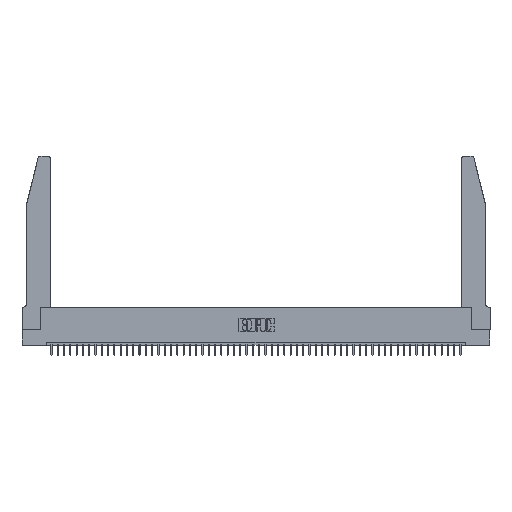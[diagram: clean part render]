
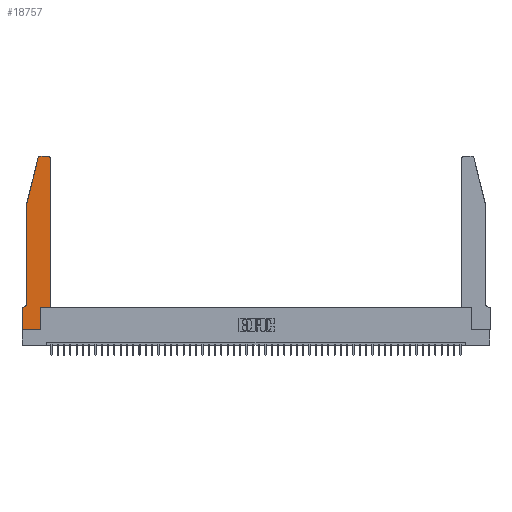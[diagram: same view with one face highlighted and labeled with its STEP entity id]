
A CAD part, top view. The second image highlights one B-rep face of the part: STEP entity #18757.
In plain terms, the highlighted planar face has unit normal (0, 0, 1).
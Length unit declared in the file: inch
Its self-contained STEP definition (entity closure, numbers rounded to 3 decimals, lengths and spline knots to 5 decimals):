
#239 = EDGE_CURVE ( 'NONE', #17133, #3528, #24382, .T. ) ;
#579 = ORIENTED_EDGE ( 'NONE', *, *, #7170, .T. ) ;
#968 = VECTOR ( 'NONE', #34424, 39.37008 ) ;
#1451 = DIRECTION ( 'NONE',  ( 0., -1., 0. ) ) ;
#2596 = ORIENTED_EDGE ( 'NONE', *, *, #239, .T. ) ;
#2757 = EDGE_CURVE ( 'NONE', #3528, #3421, #14084, .T. ) ;
#3236 = ORIENTED_EDGE ( 'NONE', *, *, #50966, .T. ) ;
#3421 = VERTEX_POINT ( 'NONE', #10675 ) ;
#3528 = VERTEX_POINT ( 'NONE', #52247 ) ;
#3619 = CARTESIAN_POINT ( 'NONE',  ( 0.4205, 2.72, 0.37 ) ) ;
#4620 = CARTESIAN_POINT ( 'NONE',  ( 0.2865, 0.35, 0.37 ) ) ;
#5196 = LINE ( 'NONE', #27130, #45272 ) ;
#5522 = CARTESIAN_POINT ( 'NONE',  ( 0.0055, 0.42, 0.37 ) ) ;
#5592 = VECTOR ( 'NONE', #7204, 39.37008 ) ;
#5607 = DIRECTION ( 'NONE',  ( -1., 0., 0. ) ) ;
#5769 = CIRCLE ( 'NONE', #48783, 0.03 ) ;
#6192 = CARTESIAN_POINT ( 'NONE',  ( 0.0755, 2., 0.37 ) ) ;
#6992 = VECTOR ( 'NONE', #36110, 39.37008 ) ;
#7170 = EDGE_CURVE ( 'NONE', #42297, #19794, #5196, .T. ) ;
#7204 = DIRECTION ( 'NONE',  ( 0., 1., 0. ) ) ;
#7736 = EDGE_CURVE ( 'NONE', #19794, #12716, #29137, .T. ) ;
#7805 = DIRECTION ( 'NONE',  ( 1., 0., 0. ) ) ;
#9256 = VERTEX_POINT ( 'NONE', #20116 ) ;
#9715 = DIRECTION ( 'NONE',  ( -1., 0., 0. ) ) ;
#10080 = DIRECTION ( 'NONE',  ( 0., 0., 1. ) ) ;
#10675 = CARTESIAN_POINT ( 'NONE',  ( 0.0755, 0.42, 0.37 ) ) ;
#10941 = CARTESIAN_POINT ( 'NONE',  ( 0.284, 2.72, 0.37 ) ) ;
#12716 = VERTEX_POINT ( 'NONE', #38595 ) ;
#12789 = VECTOR ( 'NONE', #18734, 39.37008 ) ;
#12966 = VECTOR ( 'NONE', #5607, 39.37008 ) ;
#13414 = VECTOR ( 'NONE', #52285, 39.37008 ) ;
#13481 = CARTESIAN_POINT ( 'NONE',  ( 0.4505, 0.35, 0.37 ) ) ;
#14084 = LINE ( 'NONE', #6192, #12789 ) ;
#14980 = AXIS2_PLACEMENT_3D ( 'NONE', #5522, #34498, #9715 ) ;
#15116 = DIRECTION ( 'NONE',  ( 1., 0., 0. ) ) ;
#15310 = EDGE_CURVE ( 'NONE', #9256, #40806, #22647, .T. ) ;
#15938 = CARTESIAN_POINT ( 'NONE',  ( 0., 0.35, 0.37 ) ) ;
#16922 = ORIENTED_EDGE ( 'NONE', *, *, #2757, .T. ) ;
#17133 = VERTEX_POINT ( 'NONE', #32875 ) ;
#18734 = DIRECTION ( 'NONE',  ( 0., -1., 0. ) ) ;
#18757 = ADVANCED_FACE ( 'NONE', ( #24942 ), #26548, .T. ) ;
#19310 = CARTESIAN_POINT ( 'NONE',  ( 0.2865, 0., 0.37 ) ) ;
#19583 = VERTEX_POINT ( 'NONE', #44300 ) ;
#19794 = VERTEX_POINT ( 'NONE', #13481 ) ;
#20116 = CARTESIAN_POINT ( 'NONE',  ( 0.4205, 2.75, 0.37 ) ) ;
#20121 = ORIENTED_EDGE ( 'NONE', *, *, #49427, .T. ) ;
#20726 = ORIENTED_EDGE ( 'NONE', *, *, #30848, .T. ) ;
#21307 = EDGE_LOOP ( 'NONE', ( #24708, #29857, #2596, #16922, #3236, #24000, #20121, #20726, #37521, #579, #32359, #46459 ) ) ;
#21375 = EDGE_CURVE ( 'NONE', #40806, #17133, #5769, .T. ) ;
#22647 = LINE ( 'NONE', #34583, #12966 ) ;
#22753 = DIRECTION ( 'NONE',  ( 0., 1., 0. ) ) ;
#23027 = LINE ( 'NONE', #30447, #43660 ) ;
#23273 = AXIS2_PLACEMENT_3D ( 'NONE', #3619, #32618, #7805 ) ;
#24000 = ORIENTED_EDGE ( 'NONE', *, *, #49415, .T. ) ;
#24382 = LINE ( 'NONE', #35837, #13414 ) ;
#24708 = ORIENTED_EDGE ( 'NONE', *, *, #15310, .T. ) ;
#24942 = FACE_OUTER_BOUND ( 'NONE', #21307, .T. ) ;
#26548 = PLANE ( 'NONE',  #36709 ) ;
#27130 = CARTESIAN_POINT ( 'NONE',  ( 0.4505, 0.35, 0.37 ) ) ;
#27231 = EDGE_CURVE ( 'NONE', #12716, #9256, #37071, .T. ) ;
#27850 = CARTESIAN_POINT ( 'NONE',  ( 0.2865, 0.35, 0.37 ) ) ;
#29137 = LINE ( 'NONE', #35053, #50620 ) ;
#29857 = ORIENTED_EDGE ( 'NONE', *, *, #21375, .T. ) ;
#30281 = CARTESIAN_POINT ( 'NONE',  ( 0.0755, 0.35, 0.37 ) ) ;
#30447 = CARTESIAN_POINT ( 'NONE',  ( 0., 0., 0.37 ) ) ;
#30701 = CARTESIAN_POINT ( 'NONE',  ( 0., 0.35, 0.37 ) ) ;
#30848 = EDGE_CURVE ( 'NONE', #19583, #51218, #52118, .T. ) ;
#31283 = DIRECTION ( 'NONE',  ( 1., 0., 0. ) ) ;
#31354 = VERTEX_POINT ( 'NONE', #43969 ) ;
#32359 = ORIENTED_EDGE ( 'NONE', *, *, #7736, .T. ) ;
#32618 = DIRECTION ( 'NONE',  ( 0., 0., 1. ) ) ;
#32875 = CARTESIAN_POINT ( 'NONE',  ( 0.25487, 2.72718, 0.37 ) ) ;
#34424 = DIRECTION ( 'NONE',  ( -1., 0., 0. ) ) ;
#34495 = CIRCLE ( 'NONE', #14980, 0.07 ) ;
#34498 = DIRECTION ( 'NONE',  ( 0., 0., -1. ) ) ;
#34583 = CARTESIAN_POINT ( 'NONE',  ( 0.2605, 2.75, 0.37 ) ) ;
#35053 = CARTESIAN_POINT ( 'NONE',  ( 0.4505, 0.35, 0.37 ) ) ;
#35837 = CARTESIAN_POINT ( 'NONE',  ( 0.0755, 2., 0.37 ) ) ;
#36110 = DIRECTION ( 'NONE',  ( 1., 0., 0. ) ) ;
#36616 = CARTESIAN_POINT ( 'NONE',  ( 0.284, 2.75, 0.37 ) ) ;
#36709 = AXIS2_PLACEMENT_3D ( 'NONE', #30701, #10080, #38972 ) ;
#37071 = CIRCLE ( 'NONE', #23273, 0.03 ) ;
#37316 = LINE ( 'NONE', #27850, #5592 ) ;
#37521 = ORIENTED_EDGE ( 'NONE', *, *, #48341, .T. ) ;
#38595 = CARTESIAN_POINT ( 'NONE',  ( 0.4505, 2.72, 0.37 ) ) ;
#38972 = DIRECTION ( 'NONE',  ( 1., 0., 0. ) ) ;
#39839 = DIRECTION ( 'NONE',  ( 0., 0., 1. ) ) ;
#40070 = CARTESIAN_POINT ( 'NONE',  ( 0., 0., 0.37 ) ) ;
#40806 = VERTEX_POINT ( 'NONE', #36616 ) ;
#42297 = VERTEX_POINT ( 'NONE', #4620 ) ;
#43660 = VECTOR ( 'NONE', #1451, 39.37008 ) ;
#43969 = CARTESIAN_POINT ( 'NONE',  ( 0.0055, 0.35, 0.37 ) ) ;
#44300 = CARTESIAN_POINT ( 'NONE',  ( 0., 0., 0.37 ) ) ;
#44953 = LINE ( 'NONE', #30281, #968 ) ;
#45272 = VECTOR ( 'NONE', #31283, 39.37008 ) ;
#46459 = ORIENTED_EDGE ( 'NONE', *, *, #27231, .T. ) ;
#48341 = EDGE_CURVE ( 'NONE', #51218, #42297, #37316, .T. ) ;
#48393 = VERTEX_POINT ( 'NONE', #15938 ) ;
#48783 = AXIS2_PLACEMENT_3D ( 'NONE', #10941, #39839, #15116 ) ;
#49415 = EDGE_CURVE ( 'NONE', #31354, #48393, #44953, .T. ) ;
#49427 = EDGE_CURVE ( 'NONE', #48393, #19583, #23027, .T. ) ;
#50620 = VECTOR ( 'NONE', #22753, 39.37008 ) ;
#50966 = EDGE_CURVE ( 'NONE', #3421, #31354, #34495, .T. ) ;
#51218 = VERTEX_POINT ( 'NONE', #19310 ) ;
#52118 = LINE ( 'NONE', #40070, #6992 ) ;
#52247 = CARTESIAN_POINT ( 'NONE',  ( 0.0755, 2., 0.37 ) ) ;
#52285 = DIRECTION ( 'NONE',  ( -0.239, -0.971, 0. ) ) ;
